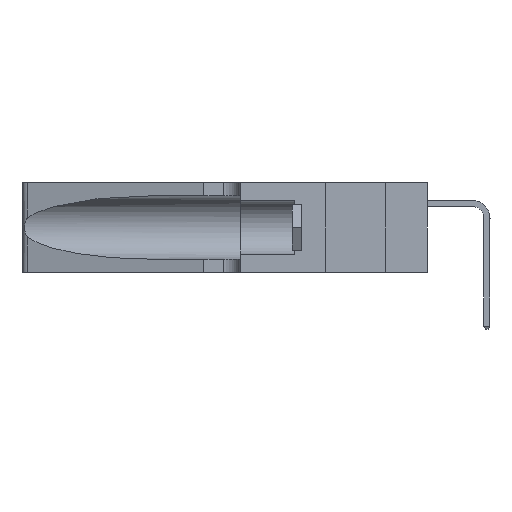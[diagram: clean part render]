
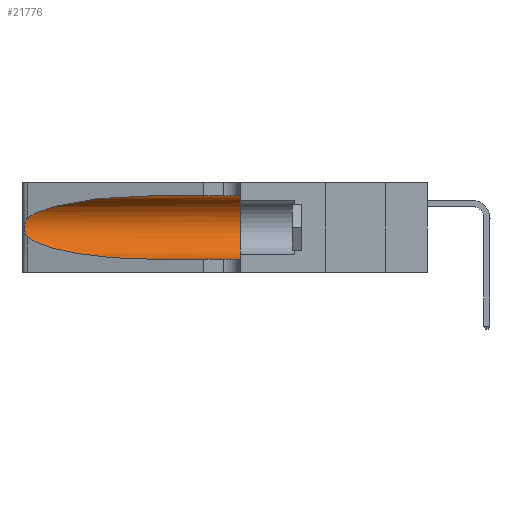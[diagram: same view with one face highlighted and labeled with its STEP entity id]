
A CAD part, left-side view. The second image highlights one B-rep face of the part: STEP entity #21776.
In plain terms, the highlighted cylindrical face has radius 3.308 mm (diameter 6.617 mm), a partial arc.
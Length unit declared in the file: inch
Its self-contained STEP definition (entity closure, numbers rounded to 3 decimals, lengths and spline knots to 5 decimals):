
#86 = AXIS2_PLACEMENT_3D ( 'NONE', #18215, #37649, #21419 ) ;
#709 = CARTESIAN_POINT ( 'NONE',  ( 0.1305, 0.72297, 0.05475 ) ) ;
#933 =( BOUNDED_CURVE ( )  B_SPLINE_CURVE ( 3, ( #21347, #37578, #11713, #2068 ),
 .UNSPECIFIED., .F., .F. ) 
 B_SPLINE_CURVE_WITH_KNOTS ( ( 4, 4 ),
 ( 3.44316, 4.71239 ),
 .UNSPECIFIED. ) 
 CURVE ( )  GEOMETRIC_REPRESENTATION_ITEM ( )  RATIONAL_B_SPLINE_CURVE ( ( 1., 0.87, 0.87, 1. ) ) 
 REPRESENTATION_ITEM ( '' )  );
#1147 = ORIENTED_EDGE ( 'NONE', *, *, #31626, .T. ) ;
#1445 = CARTESIAN_POINT ( 'NONE',  ( 0.25639, 1.23186, 0.15144 ) ) ;
#1987 = ORIENTED_EDGE ( 'NONE', *, *, #25195, .F. ) ;
#2068 = CARTESIAN_POINT ( 'NONE',  ( 0.1305, 0.72297, 0.05475 ) ) ;
#2440 = EDGE_LOOP ( 'NONE', ( #20745, #1147, #30089, #25831, #1987, #11060 ) ) ;
#2609 = VECTOR ( 'NONE', #27452, 39.37008 ) ;
#4395 = EDGE_CURVE ( 'NONE', #21124, #20944, #933, .T. ) ;
#4747 = CARTESIAN_POINT ( 'NONE',  ( 0.25487, 1.22718, 0.14631 ) ) ;
#6144 = CARTESIAN_POINT ( 'NONE',  ( 0.1305, 0.35, 0.05475 ) ) ;
#7856 = CARTESIAN_POINT ( 'NONE',  ( 0.25639, 1.23184, 0.21858 ) ) ;
#8140 = CARTESIAN_POINT ( 'NONE',  ( 0.25487, 1.22718, 0.14631 ) ) ;
#8586 = CARTESIAN_POINT ( 'NONE',  ( 0.2373, 1.15595, 0.28018 ) ) ;
#8792 = DIRECTION ( 'NONE',  ( 0., 1., 0. ) ) ;
#10819 = B_SPLINE_CURVE_WITH_KNOTS ( 'NONE', 3,
 ( #23860, #27103, #7856, #30388, #11124, #33679, #14330, #36974, #17549, #40243, #20761, #1445, #23997, #4747 ),
 .UNSPECIFIED., .F., .F.,
 ( 4, 2, 2, 2, 2, 2, 4 ),
 ( 0., 0.00027, 0.00053, 0.00107, 0.0016, 0.00187, 0.00214 ),
 .UNSPECIFIED. ) ;
#11060 = ORIENTED_EDGE ( 'NONE', *, *, #12930, .F. ) ;
#11124 = CARTESIAN_POINT ( 'NONE',  ( 0.25854, 1.2359, 0.20912 ) ) ;
#11476 = CARTESIAN_POINT ( 'NONE',  ( 0.25487, 1.22718, 0.22369 ) ) ;
#11687 = CARTESIAN_POINT ( 'NONE',  ( 0.18966, 0.96281, 0.31525 ) ) ;
#11713 = CARTESIAN_POINT ( 'NONE',  ( 0.18966, 0.96281, 0.05475 ) ) ;
#11858 = EDGE_CURVE ( 'NONE', #41494, #25111, #31321, .T. ) ;
#12375 = VECTOR ( 'NONE', #32455, 39.37008 ) ;
#12930 = EDGE_CURVE ( 'NONE', #41494, #21054, #28301, .T. ) ;
#13777 = AXIS2_PLACEMENT_3D ( 'NONE', #28022, #8792, #31309 ) ;
#14330 = CARTESIAN_POINT ( 'NONE',  ( 0.26075, 1.23896, 0.19203 ) ) ;
#17549 = CARTESIAN_POINT ( 'NONE',  ( 0.26017, 1.23833, 0.17102 ) ) ;
#17806 = VERTEX_POINT ( 'NONE', #6144 ) ;
#18215 = CARTESIAN_POINT ( 'NONE',  ( 0.1305, 1.61858, 0.185 ) ) ;
#20190 = EDGE_CURVE ( 'NONE', #20944, #17806, #28437, .T. ) ;
#20745 = ORIENTED_EDGE ( 'NONE', *, *, #11858, .T. ) ;
#20761 = CARTESIAN_POINT ( 'NONE',  ( 0.25789, 1.23486, 0.15765 ) ) ;
#20944 = VERTEX_POINT ( 'NONE', #709 ) ;
#20961 = CARTESIAN_POINT ( 'NONE',  ( 0.1305, 1.61858, 0.31525 ) ) ;
#21054 = VERTEX_POINT ( 'NONE', #23714 ) ;
#21124 = VERTEX_POINT ( 'NONE', #8140 ) ;
#21347 = CARTESIAN_POINT ( 'NONE',  ( 0.25487, 1.22718, 0.14631 ) ) ;
#21419 = DIRECTION ( 'NONE',  ( 0., 0., -1. ) ) ;
#21776 = ADVANCED_FACE ( 'NONE', ( #32388 ), #31368, .F. ) ;
#23114 = CARTESIAN_POINT ( 'NONE',  ( 0.1305, 0.72297, 0.31525 ) ) ;
#23499 = CIRCLE ( 'NONE', #13777, 0.13025 ) ;
#23714 = CARTESIAN_POINT ( 'NONE',  ( 0.1305, 0.35, 0.31525 ) ) ;
#23860 = CARTESIAN_POINT ( 'NONE',  ( 0.25487, 1.22718, 0.22369 ) ) ;
#23997 = CARTESIAN_POINT ( 'NONE',  ( 0.25555, 1.22993, 0.14849 ) ) ;
#25111 = VERTEX_POINT ( 'NONE', #11476 ) ;
#25195 = EDGE_CURVE ( 'NONE', #21054, #17806, #23499, .T. ) ;
#25831 = ORIENTED_EDGE ( 'NONE', *, *, #20190, .T. ) ;
#27103 = CARTESIAN_POINT ( 'NONE',  ( 0.25555, 1.22994, 0.2215 ) ) ;
#27452 = DIRECTION ( 'NONE',  ( 0., -1., 0. ) ) ;
#27833 = CARTESIAN_POINT ( 'NONE',  ( 0.1305, 0.72297, 0.31525 ) ) ;
#28022 = CARTESIAN_POINT ( 'NONE',  ( 0.1305, 0.35, 0.185 ) ) ;
#28301 = LINE ( 'NONE', #20961, #2609 ) ;
#28437 = LINE ( 'NONE', #29147, #12375 ) ;
#29147 = CARTESIAN_POINT ( 'NONE',  ( 0.1305, 1.61858, 0.05475 ) ) ;
#30089 = ORIENTED_EDGE ( 'NONE', *, *, #4395, .T. ) ;
#30388 = CARTESIAN_POINT ( 'NONE',  ( 0.25787, 1.23484, 0.2124 ) ) ;
#31114 = CARTESIAN_POINT ( 'NONE',  ( 0.25487, 1.22718, 0.22369 ) ) ;
#31309 = DIRECTION ( 'NONE',  ( 0., 0., 1. ) ) ;
#31321 =( BOUNDED_CURVE ( )  B_SPLINE_CURVE ( 3, ( #27833, #11687, #8586, #31114 ),
 .UNSPECIFIED., .F., .F. ) 
 B_SPLINE_CURVE_WITH_KNOTS ( ( 4, 4 ),
 ( 1.5708, 2.84003 ),
 .UNSPECIFIED. ) 
 CURVE ( )  GEOMETRIC_REPRESENTATION_ITEM ( )  RATIONAL_B_SPLINE_CURVE ( ( 1., 0.87, 0.87, 1. ) ) 
 REPRESENTATION_ITEM ( '' )  );
#31368 = CYLINDRICAL_SURFACE ( 'NONE', #86, 0.13025 ) ;
#31626 = EDGE_CURVE ( 'NONE', #25111, #21124, #10819, .T. ) ;
#32388 = FACE_OUTER_BOUND ( 'NONE', #2440, .T. ) ;
#32455 = DIRECTION ( 'NONE',  ( 0., -1., 0. ) ) ;
#33679 = CARTESIAN_POINT ( 'NONE',  ( 0.26018, 1.23835, 0.19895 ) ) ;
#36974 = CARTESIAN_POINT ( 'NONE',  ( 0.26075, 1.23896, 0.178 ) ) ;
#37578 = CARTESIAN_POINT ( 'NONE',  ( 0.2373, 1.15595, 0.08982 ) ) ;
#37649 = DIRECTION ( 'NONE',  ( 0., -1., 0. ) ) ;
#40243 = CARTESIAN_POINT ( 'NONE',  ( 0.25856, 1.23593, 0.16098 ) ) ;
#41494 = VERTEX_POINT ( 'NONE', #23114 ) ;
